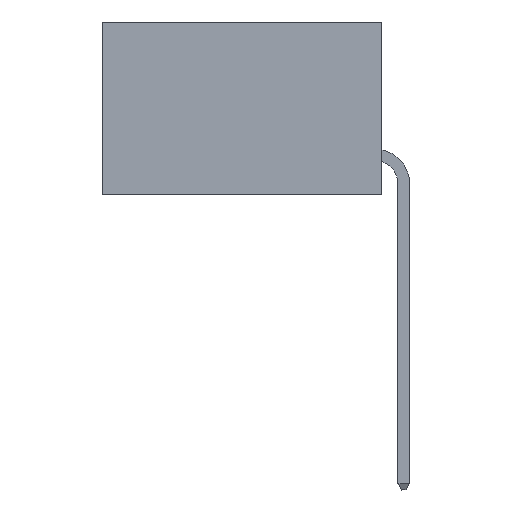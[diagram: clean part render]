
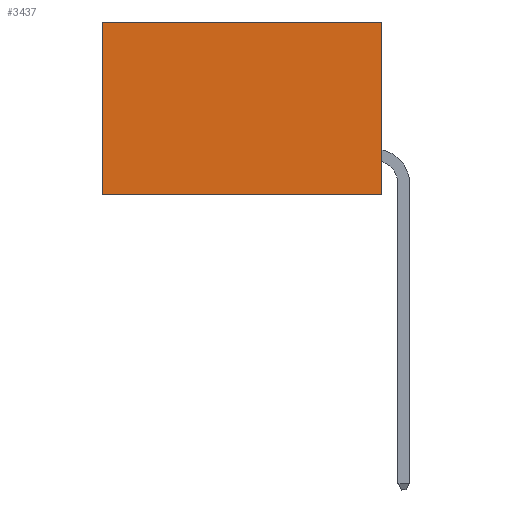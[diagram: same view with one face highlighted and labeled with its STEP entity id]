
A CAD part, left-side view. The second image highlights one B-rep face of the part: STEP entity #3437.
In plain terms, the highlighted planar face has unit normal (-1, 0, 0).
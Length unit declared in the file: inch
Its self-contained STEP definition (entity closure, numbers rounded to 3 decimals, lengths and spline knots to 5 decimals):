
#4 = EDGE_CURVE ( 'NONE', #7671, #5031, #26, .T. ) ;
#26 = LINE ( 'NONE', #1544, #5958 ) ;
#38 = CARTESIAN_POINT ( 'NONE',  ( 0.2875, 0., -0.37 ) ) ;
#691 = DIRECTION ( 'NONE',  ( 1., 0., 0. ) ) ;
#1377 = DIRECTION ( 'NONE',  ( 0., 0., -1. ) ) ;
#1544 = CARTESIAN_POINT ( 'NONE',  ( 0.2875, 0.6, 0. ) ) ;
#1643 = LINE ( 'NONE', #2604, #4528 ) ;
#2198 = VECTOR ( 'NONE', #4663, 39.37008 ) ;
#2322 = CARTESIAN_POINT ( 'NONE',  ( 0.2875, 0.6, 0. ) ) ;
#2475 = CARTESIAN_POINT ( 'NONE',  ( 0.2875, 0., 0. ) ) ;
#2604 = CARTESIAN_POINT ( 'NONE',  ( 0.2875, 0., 0. ) ) ;
#2874 = CARTESIAN_POINT ( 'NONE',  ( 0.2875, 0.6, -0.37 ) ) ;
#3064 = FACE_OUTER_BOUND ( 'NONE', #6321, .T. ) ;
#3194 = LINE ( 'NONE', #38, #2198 ) ;
#3300 = EDGE_CURVE ( 'NONE', #5523, #7671, #8078, .T. ) ;
#3341 = ORIENTED_EDGE ( 'NONE', *, *, #4, .T. ) ;
#3363 = CARTESIAN_POINT ( 'NONE',  ( 0.2875, 0., -0.37 ) ) ;
#3437 = ADVANCED_FACE ( 'NONE', ( #3064 ), #5280, .F. ) ;
#3503 = EDGE_CURVE ( 'NONE', #5523, #6187, #1643, .T. ) ;
#3805 = DIRECTION ( 'NONE',  ( 0., 1., 0. ) ) ;
#3885 = ORIENTED_EDGE ( 'NONE', *, *, #3300, .T. ) ;
#3888 = VECTOR ( 'NONE', #3805, 39.37008 ) ;
#4088 = ORIENTED_EDGE ( 'NONE', *, *, #6197, .F. ) ;
#4333 = AXIS2_PLACEMENT_3D ( 'NONE', #4637, #691, #1377 ) ;
#4528 = VECTOR ( 'NONE', #8544, 39.37008 ) ;
#4637 = CARTESIAN_POINT ( 'NONE',  ( 0.2875, 0., 0. ) ) ;
#4663 = DIRECTION ( 'NONE',  ( 0., 1., 0. ) ) ;
#4901 = DIRECTION ( 'NONE',  ( 0., 0., -1. ) ) ;
#5031 = VERTEX_POINT ( 'NONE', #2874 ) ;
#5133 = ORIENTED_EDGE ( 'NONE', *, *, #3503, .F. ) ;
#5280 = PLANE ( 'NONE',  #4333 ) ;
#5523 = VERTEX_POINT ( 'NONE', #5926 ) ;
#5926 = CARTESIAN_POINT ( 'NONE',  ( 0.2875, 0., 0. ) ) ;
#5958 = VECTOR ( 'NONE', #4901, 39.37008 ) ;
#6187 = VERTEX_POINT ( 'NONE', #3363 ) ;
#6197 = EDGE_CURVE ( 'NONE', #6187, #5031, #3194, .T. ) ;
#6321 = EDGE_LOOP ( 'NONE', ( #3341, #4088, #5133, #3885 ) ) ;
#7671 = VERTEX_POINT ( 'NONE', #2322 ) ;
#8078 = LINE ( 'NONE', #2475, #3888 ) ;
#8544 = DIRECTION ( 'NONE',  ( 0., 0., -1. ) ) ;
